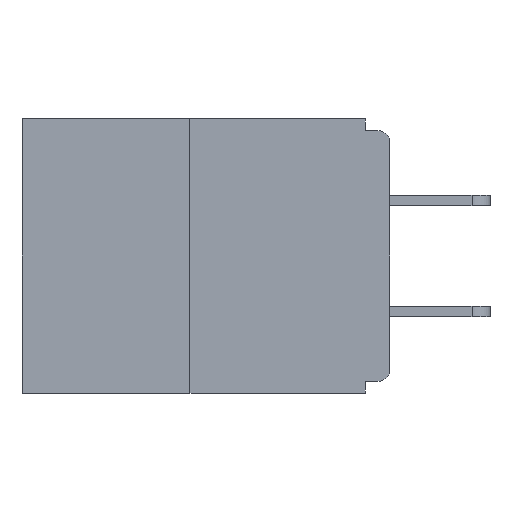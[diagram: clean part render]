
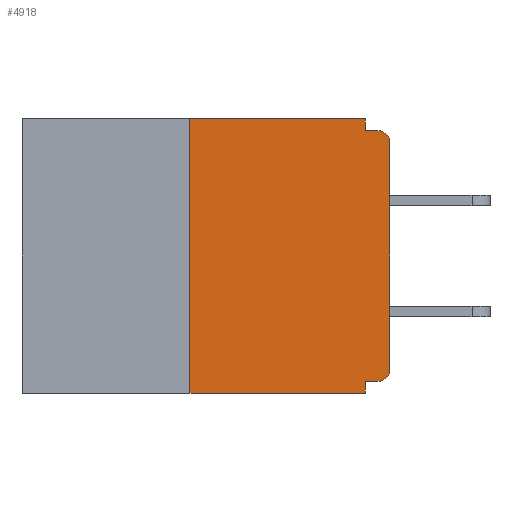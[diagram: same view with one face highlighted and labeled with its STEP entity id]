
A CAD part, left-side view. The second image highlights one B-rep face of the part: STEP entity #4918.
In plain terms, the highlighted planar face has unit normal (-1, 0, 0).
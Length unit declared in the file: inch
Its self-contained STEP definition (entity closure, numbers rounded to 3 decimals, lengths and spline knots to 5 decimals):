
#405 = ORIENTED_EDGE ( 'NONE', *, *, #1422, .F. ) ;
#902 = EDGE_CURVE ( 'NONE', #20112, #14093, #22796, .T. ) ;
#965 = CARTESIAN_POINT ( 'NONE',  ( 0., 0.031, 0. ) ) ;
#1369 = FACE_OUTER_BOUND ( 'NONE', #19411, .T. ) ;
#1422 = EDGE_CURVE ( 'NONE', #27874, #4912, #27965, .T. ) ;
#1708 = CARTESIAN_POINT ( 'NONE',  ( 0., 0.015, -0.015 ) ) ;
#2076 = EDGE_CURVE ( 'NONE', #14093, #22809, #26308, .T. ) ;
#2395 = VERTEX_POINT ( 'NONE', #15749 ) ;
#2793 = DIRECTION ( 'NONE',  ( 0., -1., 0. ) ) ;
#3363 = VECTOR ( 'NONE', #18637, 39.37008 ) ;
#3618 = CARTESIAN_POINT ( 'NONE',  ( 0., 0.031, -0.328 ) ) ;
#3710 = PLANE ( 'NONE',  #16462 ) ;
#3813 = CARTESIAN_POINT ( 'NONE',  ( 0., 0.015, -0.313 ) ) ;
#4056 = CARTESIAN_POINT ( 'NONE',  ( 0., 0.031, -0.015 ) ) ;
#4367 = CARTESIAN_POINT ( 'NONE',  ( 0., 0.015, -0.03 ) ) ;
#4459 = ORIENTED_EDGE ( 'NONE', *, *, #25590, .F. ) ;
#4912 = VERTEX_POINT ( 'NONE', #3618 ) ;
#4918 = ADVANCED_FACE ( 'NONE', ( #1369 ), #3710, .F. ) ;
#5298 = CARTESIAN_POINT ( 'NONE',  ( 0., 0.031, 0. ) ) ;
#5577 = ORIENTED_EDGE ( 'NONE', *, *, #23696, .F. ) ;
#5824 = CARTESIAN_POINT ( 'NONE',  ( 0., 0., 0. ) ) ;
#5936 = VECTOR ( 'NONE', #8511, 39.37008 ) ;
#6001 = DIRECTION ( 'NONE',  ( 0., 0., -1. ) ) ;
#6263 = CARTESIAN_POINT ( 'NONE',  ( 0., 0.46, -0.343 ) ) ;
#6390 = DIRECTION ( 'NONE',  ( 0., 0., 1. ) ) ;
#6507 = ORIENTED_EDGE ( 'NONE', *, *, #14001, .T. ) ;
#6637 = VECTOR ( 'NONE', #6390, 39.37008 ) ;
#6826 = CARTESIAN_POINT ( 'NONE',  ( 0., 0.25, -0.343 ) ) ;
#6892 = VECTOR ( 'NONE', #10568, 39.37008 ) ;
#7650 = ORIENTED_EDGE ( 'NONE', *, *, #13441, .T. ) ;
#8432 = CARTESIAN_POINT ( 'NONE',  ( 0., 0., -0.015 ) ) ;
#8475 = VECTOR ( 'NONE', #12951, 39.37008 ) ;
#8483 = DIRECTION ( 'NONE',  ( 0., -1., 0. ) ) ;
#8511 = DIRECTION ( 'NONE',  ( 0., 1., 0. ) ) ;
#8709 = ORIENTED_EDGE ( 'NONE', *, *, #11641, .F. ) ;
#8992 = VERTEX_POINT ( 'NONE', #965 ) ;
#9168 = DIRECTION ( 'NONE',  ( -1., 0., 0. ) ) ;
#9411 = ORIENTED_EDGE ( 'NONE', *, *, #14116, .F. ) ;
#10049 = DIRECTION ( 'NONE',  ( 1., 0., 0. ) ) ;
#10413 = CARTESIAN_POINT ( 'NONE',  ( 0., 0., -0.313 ) ) ;
#10568 = DIRECTION ( 'NONE',  ( 0., 0., -1. ) ) ;
#11641 = EDGE_CURVE ( 'NONE', #17155, #22809, #12607, .T. ) ;
#12093 = CIRCLE ( 'NONE', #26414, 0.015 ) ;
#12468 = VECTOR ( 'NONE', #8483, 39.37008 ) ;
#12560 = CARTESIAN_POINT ( 'NONE',  ( 0., 0.031, -0.343 ) ) ;
#12607 = LINE ( 'NONE', #8432, #8475 ) ;
#12951 = DIRECTION ( 'NONE',  ( 0., -1., 0. ) ) ;
#13441 = EDGE_CURVE ( 'NONE', #13641, #15433, #14534, .T. ) ;
#13641 = VERTEX_POINT ( 'NONE', #6826 ) ;
#14001 = EDGE_CURVE ( 'NONE', #27874, #20112, #12093, .T. ) ;
#14093 = VERTEX_POINT ( 'NONE', #14319 ) ;
#14116 = EDGE_CURVE ( 'NONE', #8992, #17155, #26547, .T. ) ;
#14166 = VECTOR ( 'NONE', #22783, 39.37008 ) ;
#14319 = CARTESIAN_POINT ( 'NONE',  ( 0., 0., -0.03 ) ) ;
#14498 = CARTESIAN_POINT ( 'NONE',  ( 0., 0.25, 0. ) ) ;
#14534 = LINE ( 'NONE', #6263, #12468 ) ;
#15433 = VERTEX_POINT ( 'NONE', #12560 ) ;
#15749 = CARTESIAN_POINT ( 'NONE',  ( 0., 0.25, 0. ) ) ;
#15778 = DIRECTION ( 'NONE',  ( 0., 0., -1. ) ) ;
#16064 = CARTESIAN_POINT ( 'NONE',  ( 0., 0.015, -0.328 ) ) ;
#16462 = AXIS2_PLACEMENT_3D ( 'NONE', #25618, #10049, #21187 ) ;
#17155 = VERTEX_POINT ( 'NONE', #4056 ) ;
#17346 = CARTESIAN_POINT ( 'NONE',  ( 0., 0., -0.328 ) ) ;
#18637 = DIRECTION ( 'NONE',  ( 0., 0., 1. ) ) ;
#19171 = DIRECTION ( 'NONE',  ( -1., 0., 0. ) ) ;
#19411 = EDGE_LOOP ( 'NONE', ( #5577, #4459, #7650, #23658, #405, #6507, #27980, #21805, #8709, #9411 ) ) ;
#19623 = LINE ( 'NONE', #26910, #24099 ) ;
#19840 = LINE ( 'NONE', #14498, #3363 ) ;
#20112 = VERTEX_POINT ( 'NONE', #10413 ) ;
#20451 = AXIS2_PLACEMENT_3D ( 'NONE', #4367, #9168, #15778 ) ;
#21187 = DIRECTION ( 'NONE',  ( 0., 0., -1. ) ) ;
#21805 = ORIENTED_EDGE ( 'NONE', *, *, #2076, .T. ) ;
#22783 = DIRECTION ( 'NONE',  ( 0., 0., -1. ) ) ;
#22796 = LINE ( 'NONE', #5824, #6637 ) ;
#22809 = VERTEX_POINT ( 'NONE', #1708 ) ;
#23171 = EDGE_CURVE ( 'NONE', #4912, #15433, #23433, .T. ) ;
#23433 = LINE ( 'NONE', #23987, #6892 ) ;
#23658 = ORIENTED_EDGE ( 'NONE', *, *, #23171, .F. ) ;
#23696 = EDGE_CURVE ( 'NONE', #2395, #8992, #19623, .T. ) ;
#23987 = CARTESIAN_POINT ( 'NONE',  ( 0., 0.031, -0.343 ) ) ;
#24099 = VECTOR ( 'NONE', #2793, 39.37008 ) ;
#25590 = EDGE_CURVE ( 'NONE', #13641, #2395, #19840, .T. ) ;
#25618 = CARTESIAN_POINT ( 'NONE',  ( 0., 0.46, 0. ) ) ;
#26308 = CIRCLE ( 'NONE', #20451, 0.015 ) ;
#26414 = AXIS2_PLACEMENT_3D ( 'NONE', #3813, #19171, #6001 ) ;
#26547 = LINE ( 'NONE', #5298, #14166 ) ;
#26910 = CARTESIAN_POINT ( 'NONE',  ( 0., 0.46, 0. ) ) ;
#27874 = VERTEX_POINT ( 'NONE', #16064 ) ;
#27965 = LINE ( 'NONE', #17346, #5936 ) ;
#27980 = ORIENTED_EDGE ( 'NONE', *, *, #902, .T. ) ;
